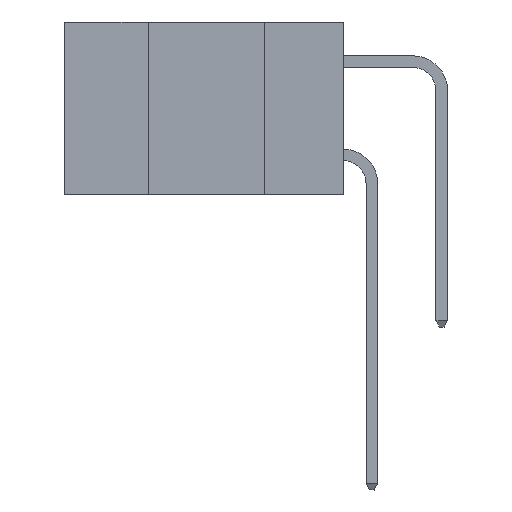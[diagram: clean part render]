
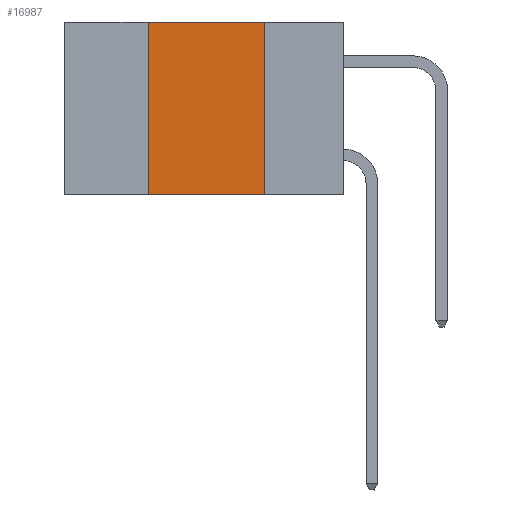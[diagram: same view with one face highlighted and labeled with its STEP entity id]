
A CAD part, left-side view. The second image highlights one B-rep face of the part: STEP entity #16987.
In plain terms, the highlighted planar face has unit normal (-1, 0, 0).
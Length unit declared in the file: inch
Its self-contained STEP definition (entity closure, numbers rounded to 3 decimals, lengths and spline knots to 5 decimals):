
#917 = AXIS2_PLACEMENT_3D ( 'NONE', #13295, #4151, #14758 ) ;
#1220 = CARTESIAN_POINT ( 'NONE',  ( 0., 0.17, -0.37 ) ) ;
#1257 = DIRECTION ( 'NONE',  ( 0., -1., 0. ) ) ;
#2232 = VECTOR ( 'NONE', #10425, 39.37008 ) ;
#2529 = LINE ( 'NONE', #1220, #12525 ) ;
#2559 = CARTESIAN_POINT ( 'NONE',  ( 0., 0.42, -0.37 ) ) ;
#2652 = VERTEX_POINT ( 'NONE', #7512 ) ;
#3072 = ORIENTED_EDGE ( 'NONE', *, *, #12350, .F. ) ;
#3102 = CARTESIAN_POINT ( 'NONE',  ( 0., 0.6, 0. ) ) ;
#3638 = LINE ( 'NONE', #7622, #2232 ) ;
#4151 = DIRECTION ( 'NONE',  ( 1., 0., 0. ) ) ;
#4918 = VERTEX_POINT ( 'NONE', #11301 ) ;
#6514 = DIRECTION ( 'NONE',  ( 0., 0., -1. ) ) ;
#7185 = DIRECTION ( 'NONE',  ( 0., -1., 0. ) ) ;
#7512 = CARTESIAN_POINT ( 'NONE',  ( 0., 0.17, -0.37 ) ) ;
#7622 = CARTESIAN_POINT ( 'NONE',  ( 0., 0.42, -0.37 ) ) ;
#7815 = ORIENTED_EDGE ( 'NONE', *, *, #12013, .F. ) ;
#8016 = EDGE_CURVE ( 'NONE', #15923, #4918, #12417, .T. ) ;
#9462 = FACE_OUTER_BOUND ( 'NONE', #12713, .T. ) ;
#10425 = DIRECTION ( 'NONE',  ( 0., 0., 1. ) ) ;
#10491 = VECTOR ( 'NONE', #7185, 39.37008 ) ;
#10564 = CARTESIAN_POINT ( 'NONE',  ( 0., 0.6, -0.37 ) ) ;
#10765 = PLANE ( 'NONE',  #917 ) ;
#11301 = CARTESIAN_POINT ( 'NONE',  ( 0., 0.17, 0. ) ) ;
#11469 = EDGE_CURVE ( 'NONE', #14699, #2652, #14563, .T. ) ;
#12013 = EDGE_CURVE ( 'NONE', #4918, #2652, #2529, .T. ) ;
#12158 = ORIENTED_EDGE ( 'NONE', *, *, #11469, .T. ) ;
#12231 = VECTOR ( 'NONE', #1257, 39.37008 ) ;
#12350 = EDGE_CURVE ( 'NONE', #14699, #15923, #3638, .T. ) ;
#12417 = LINE ( 'NONE', #3102, #10491 ) ;
#12525 = VECTOR ( 'NONE', #6514, 39.37008 ) ;
#12551 = ORIENTED_EDGE ( 'NONE', *, *, #8016, .F. ) ;
#12713 = EDGE_LOOP ( 'NONE', ( #7815, #12551, #3072, #12158 ) ) ;
#13170 = CARTESIAN_POINT ( 'NONE',  ( 0., 0.42, 0. ) ) ;
#13295 = CARTESIAN_POINT ( 'NONE',  ( 0., 0.6, 0. ) ) ;
#14563 = LINE ( 'NONE', #10564, #12231 ) ;
#14699 = VERTEX_POINT ( 'NONE', #2559 ) ;
#14758 = DIRECTION ( 'NONE',  ( 0., 0., -1. ) ) ;
#15923 = VERTEX_POINT ( 'NONE', #13170 ) ;
#16987 = ADVANCED_FACE ( 'NONE', ( #9462 ), #10765, .F. ) ;
